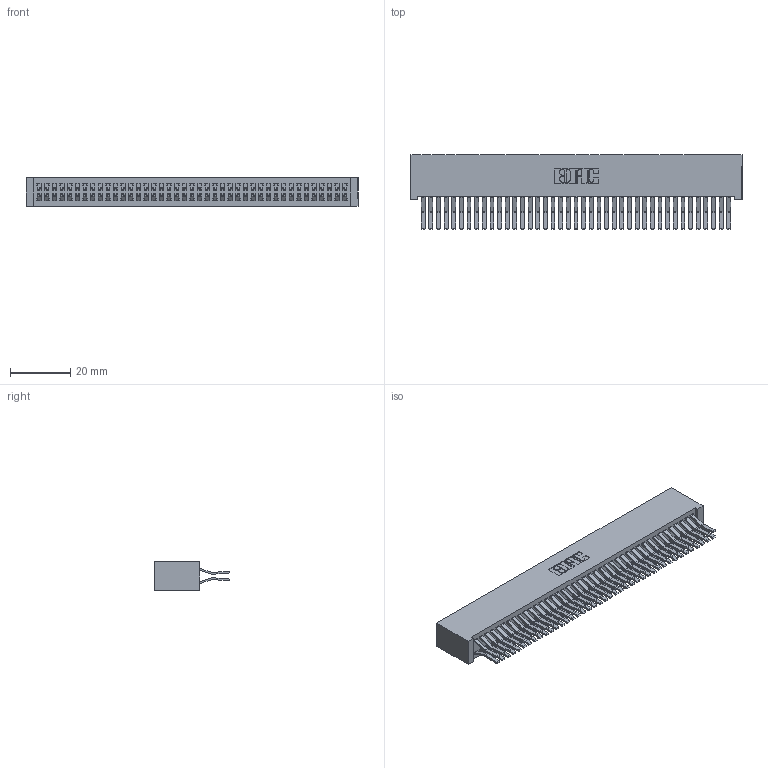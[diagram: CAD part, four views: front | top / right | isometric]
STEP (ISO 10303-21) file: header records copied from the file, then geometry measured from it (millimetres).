
FILE_DESCRIPTION (( 'STEP AP203' ), '1' );
FILE_NAME ('392-082-560-201.STEP', '2018-08-18T04:07:01', ( '' ), ( '' ), 'SwSTEP 2.0', 'SolidWorks 2016', '' );
FILE_SCHEMA (( 'CONFIG_CONTROL_DESIGN' ));
Length unit declared in the file: inch
Products named in the file (3): 342 Part_Lugless; 345-292-001_560 Tail; 392-082-560-201
Assembly tree (83 placements, depth 2):
  392-082-560-201
    342 Part_Lugless
    345-292-001_560 Tail  x82
Bounding box: 110.39 x 24.78 x 9.4 mm (x, y, z)
Volume: 10891.5 mm3; surface area: 19441.2 mm2
Topology: 83 solids, 83 shells, 4530 faces, 13477 edges, 8874 vertices
Faces by surface type: plane 3014, cylinder 1516
Entity records: 26185 total; most frequent: CARTESIAN_POINT 4338, ORIENTED_EDGE 4274, DIRECTION 3705, EDGE_CURVE 2137, VECTOR 2013, LINE 2013, VERTEX_POINT 1422, AXIS2_PLACEMENT_3D 846
